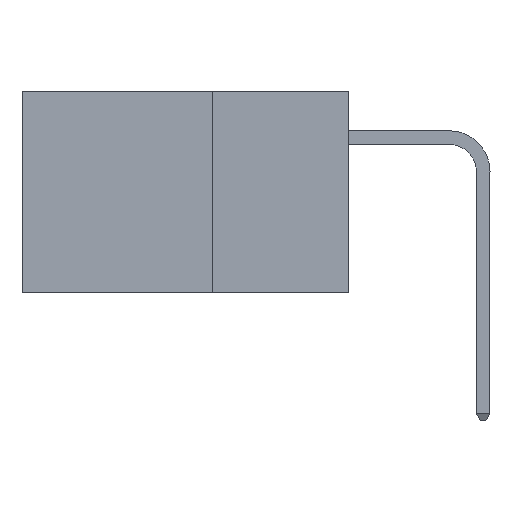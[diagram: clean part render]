
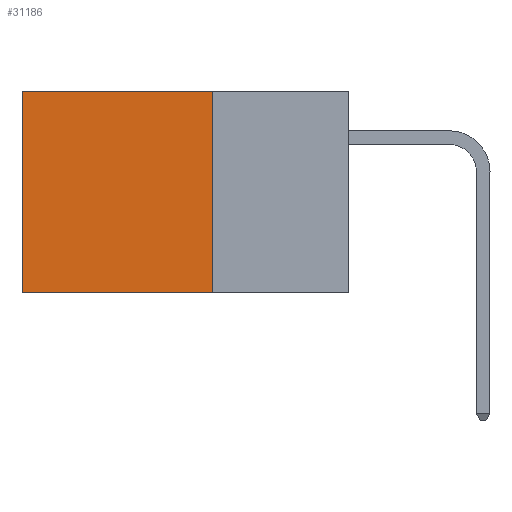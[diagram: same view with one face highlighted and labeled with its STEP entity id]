
A CAD part, left-side view. The second image highlights one B-rep face of the part: STEP entity #31186.
In plain terms, the highlighted planar face has unit normal (-1, 0, 0).
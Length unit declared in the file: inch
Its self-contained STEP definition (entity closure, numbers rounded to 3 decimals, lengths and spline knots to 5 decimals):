
#323 = ORIENTED_EDGE ( 'NONE', *, *, #4676, .F. ) ;
#2315 = VERTEX_POINT ( 'NONE', #31671 ) ;
#2316 = FACE_OUTER_BOUND ( 'NONE', #35011, .T. ) ;
#4323 = LINE ( 'NONE', #26145, #19153 ) ;
#4676 = EDGE_CURVE ( 'NONE', #2315, #23358, #28334, .T. ) ;
#7487 = CARTESIAN_POINT ( 'NONE',  ( 0.2875, 0.25, 0. ) ) ;
#7500 = CARTESIAN_POINT ( 'NONE',  ( 0.2875, 0.6, 0. ) ) ;
#7926 = EDGE_CURVE ( 'NONE', #37108, #2315, #30210, .T. ) ;
#12859 = DIRECTION ( 'NONE',  ( 0., 1., 0. ) ) ;
#13037 = CARTESIAN_POINT ( 'NONE',  ( 0.2875, 0.25, 0. ) ) ;
#14380 = CARTESIAN_POINT ( 'NONE',  ( 0.2875, 0.6, 0. ) ) ;
#16391 = PLANE ( 'NONE',  #32531 ) ;
#16918 = ORIENTED_EDGE ( 'NONE', *, *, #29704, .T. ) ;
#17350 = DIRECTION ( 'NONE',  ( 0., 0., -1. ) ) ;
#17378 = CARTESIAN_POINT ( 'NONE',  ( 0.2875, 0.25, 0. ) ) ;
#17480 = CARTESIAN_POINT ( 'NONE',  ( 0.2875, 0.6, -0.37 ) ) ;
#19153 = VECTOR ( 'NONE', #28803, 39.37008 ) ;
#19325 = DIRECTION ( 'NONE',  ( 0., 0., -1. ) ) ;
#19666 = EDGE_CURVE ( 'NONE', #29405, #23358, #21559, .T. ) ;
#20670 = VECTOR ( 'NONE', #17350, 39.37008 ) ;
#20835 = VECTOR ( 'NONE', #12859, 39.37008 ) ;
#21559 = LINE ( 'NONE', #14380, #20670 ) ;
#23358 = VERTEX_POINT ( 'NONE', #17480 ) ;
#23508 = DIRECTION ( 'NONE',  ( 0., 0., -1. ) ) ;
#26145 = CARTESIAN_POINT ( 'NONE',  ( 0.2875, 0.25, 0. ) ) ;
#27183 = CARTESIAN_POINT ( 'NONE',  ( 0.2875, 0.25, -0.37 ) ) ;
#28302 = ORIENTED_EDGE ( 'NONE', *, *, #19666, .T. ) ;
#28334 = LINE ( 'NONE', #27183, #20835 ) ;
#28803 = DIRECTION ( 'NONE',  ( 0., 1., 0. ) ) ;
#29405 = VERTEX_POINT ( 'NONE', #7500 ) ;
#29704 = EDGE_CURVE ( 'NONE', #37108, #29405, #4323, .T. ) ;
#30210 = LINE ( 'NONE', #17378, #36720 ) ;
#31186 = ADVANCED_FACE ( 'NONE', ( #2316 ), #16391, .F. ) ;
#31671 = CARTESIAN_POINT ( 'NONE',  ( 0.2875, 0.25, -0.37 ) ) ;
#32531 = AXIS2_PLACEMENT_3D ( 'NONE', #7487, #36065, #19325 ) ;
#35011 = EDGE_LOOP ( 'NONE', ( #28302, #323, #36728, #16918 ) ) ;
#36065 = DIRECTION ( 'NONE',  ( 1., 0., 0. ) ) ;
#36720 = VECTOR ( 'NONE', #23508, 39.37008 ) ;
#36728 = ORIENTED_EDGE ( 'NONE', *, *, #7926, .F. ) ;
#37108 = VERTEX_POINT ( 'NONE', #13037 ) ;
